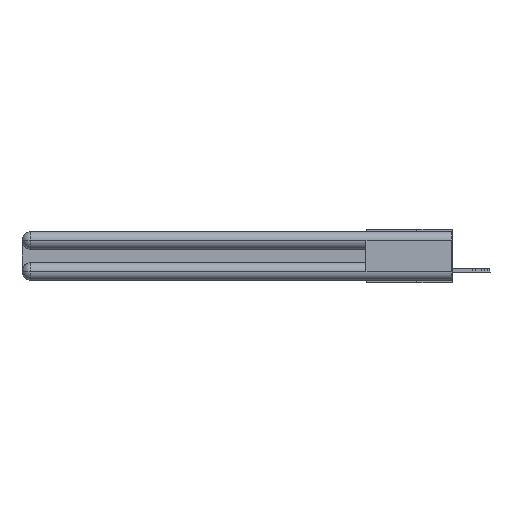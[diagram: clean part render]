
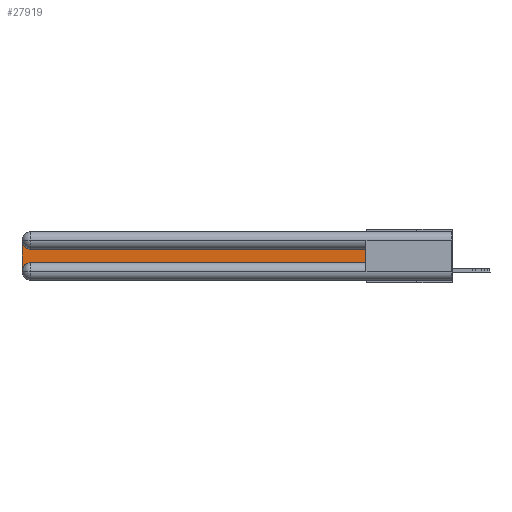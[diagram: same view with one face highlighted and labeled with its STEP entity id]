
A CAD part, left-side view. The second image highlights one B-rep face of the part: STEP entity #27919.
In plain terms, the highlighted planar face has unit normal (-1, 0, 0).
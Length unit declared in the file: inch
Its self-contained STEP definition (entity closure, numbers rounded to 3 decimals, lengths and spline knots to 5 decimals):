
#197 = EDGE_CURVE ( 'NONE', #9096, #22456, #15598, .T. ) ;
#766 = CIRCLE ( 'NONE', #1649, 0.06 ) ;
#779 = EDGE_CURVE ( 'NONE', #23222, #5506, #29283, .T. ) ;
#1649 = AXIS2_PLACEMENT_3D ( 'NONE', #25907, #4708, #18700 ) ;
#2273 = DIRECTION ( 'NONE',  ( 0., 1., 0. ) ) ;
#2351 = VERTEX_POINT ( 'NONE', #6942 ) ;
#3222 = CARTESIAN_POINT ( 'NONE',  ( 0.075, 2.94, -0.1225 ) ) ;
#4267 = ORIENTED_EDGE ( 'NONE', *, *, #779, .T. ) ;
#4708 = DIRECTION ( 'NONE',  ( 1., 0., 0. ) ) ;
#5506 = VERTEX_POINT ( 'NONE', #12307 ) ;
#5627 = DIRECTION ( 'NONE',  ( 0., -1., 0. ) ) ;
#6034 = CARTESIAN_POINT ( 'NONE',  ( 0.075, 0.6, -0.2175 ) ) ;
#6639 = DIRECTION ( 'NONE',  ( 1., 0., 0. ) ) ;
#6648 = EDGE_LOOP ( 'NONE', ( #18251, #16989, #20708, #25288, #4267, #28598 ) ) ;
#6726 = AXIS2_PLACEMENT_3D ( 'NONE', #21529, #19346, #16765 ) ;
#6942 = CARTESIAN_POINT ( 'NONE',  ( 0.075, 3., -0.0625 ) ) ;
#6972 = VECTOR ( 'NONE', #16898, 39.37008 ) ;
#9096 = VERTEX_POINT ( 'NONE', #17253 ) ;
#9154 = CIRCLE ( 'NONE', #6726, 0.06 ) ;
#12206 = AXIS2_PLACEMENT_3D ( 'NONE', #25548, #6639, #20754 ) ;
#12307 = CARTESIAN_POINT ( 'NONE',  ( 0.075, 0.6, -0.2175 ) ) ;
#13115 = EDGE_CURVE ( 'NONE', #15325, #23222, #766, .T. ) ;
#15325 = VERTEX_POINT ( 'NONE', #21570 ) ;
#15598 = LINE ( 'NONE', #21355, #26698 ) ;
#16282 = PLANE ( 'NONE',  #12206 ) ;
#16765 = DIRECTION ( 'NONE',  ( 0., 0., -1. ) ) ;
#16898 = DIRECTION ( 'NONE',  ( 0., 0., 1. ) ) ;
#16989 = ORIENTED_EDGE ( 'NONE', *, *, #21634, .T. ) ;
#17253 = CARTESIAN_POINT ( 'NONE',  ( 0.075, 0.6, -0.1225 ) ) ;
#17375 = LINE ( 'NONE', #19579, #6972 ) ;
#17932 = LINE ( 'NONE', #22229, #19749 ) ;
#18251 = ORIENTED_EDGE ( 'NONE', *, *, #197, .T. ) ;
#18700 = DIRECTION ( 'NONE',  ( 0., 0., -1. ) ) ;
#18704 = EDGE_CURVE ( 'NONE', #2351, #15325, #17932, .T. ) ;
#18912 = CARTESIAN_POINT ( 'NONE',  ( 0.075, 2.94, -0.2175 ) ) ;
#19334 = FACE_OUTER_BOUND ( 'NONE', #6648, .T. ) ;
#19346 = DIRECTION ( 'NONE',  ( 1., 0., 0. ) ) ;
#19579 = CARTESIAN_POINT ( 'NONE',  ( 0.075, 0.6, -0.2175 ) ) ;
#19749 = VECTOR ( 'NONE', #29385, 39.37008 ) ;
#20708 = ORIENTED_EDGE ( 'NONE', *, *, #18704, .T. ) ;
#20754 = DIRECTION ( 'NONE',  ( 0., 0., -1. ) ) ;
#21355 = CARTESIAN_POINT ( 'NONE',  ( 0.075, 0.6, -0.1225 ) ) ;
#21529 = CARTESIAN_POINT ( 'NONE',  ( 0.075, 2.94, -0.0625 ) ) ;
#21570 = CARTESIAN_POINT ( 'NONE',  ( 0.075, 3., -0.2775 ) ) ;
#21634 = EDGE_CURVE ( 'NONE', #22456, #2351, #9154, .T. ) ;
#22229 = CARTESIAN_POINT ( 'NONE',  ( 0.075, 3., -0.2175 ) ) ;
#22456 = VERTEX_POINT ( 'NONE', #3222 ) ;
#22970 = VECTOR ( 'NONE', #5627, 39.37008 ) ;
#23222 = VERTEX_POINT ( 'NONE', #18912 ) ;
#24023 = EDGE_CURVE ( 'NONE', #5506, #9096, #17375, .T. ) ;
#25288 = ORIENTED_EDGE ( 'NONE', *, *, #13115, .T. ) ;
#25548 = CARTESIAN_POINT ( 'NONE',  ( 0.075, 3., -0.1225 ) ) ;
#25907 = CARTESIAN_POINT ( 'NONE',  ( 0.075, 2.94, -0.2775 ) ) ;
#26698 = VECTOR ( 'NONE', #2273, 39.37008 ) ;
#27919 = ADVANCED_FACE ( 'NONE', ( #19334 ), #16282, .F. ) ;
#28598 = ORIENTED_EDGE ( 'NONE', *, *, #24023, .T. ) ;
#29283 = LINE ( 'NONE', #6034, #22970 ) ;
#29385 = DIRECTION ( 'NONE',  ( 0., 0., -1. ) ) ;
